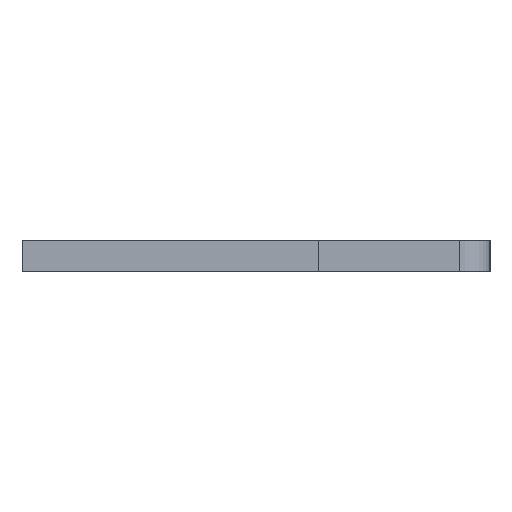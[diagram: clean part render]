
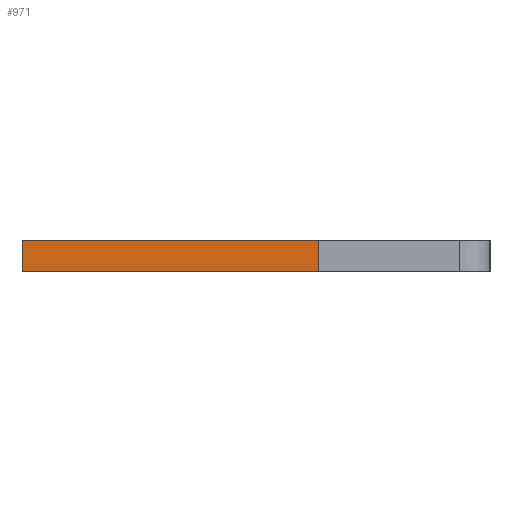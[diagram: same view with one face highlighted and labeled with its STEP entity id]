
A CAD part, left-side view. The second image highlights one B-rep face of the part: STEP entity #971.
In plain terms, the highlighted face is planar.
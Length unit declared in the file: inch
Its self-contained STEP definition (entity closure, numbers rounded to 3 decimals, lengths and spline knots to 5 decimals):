
#16 = LINE ( 'NONE', #1397, #754 ) ;
#61 = ORIENTED_EDGE ( 'NONE', *, *, #1215, .F. ) ;
#216 = ORIENTED_EDGE ( 'NONE', *, *, #1568, .F. ) ;
#306 = CARTESIAN_POINT ( 'NONE',  ( 0.01, 0.15, -0.04 ) ) ;
#328 = CARTESIAN_POINT ( 'NONE',  ( 0.01, 0.15, -0.04 ) ) ;
#353 = VECTOR ( 'NONE', #358, 39.37008 ) ;
#358 = DIRECTION ( 'NONE',  ( -1., 0., 0. ) ) ;
#361 = VERTEX_POINT ( 'NONE', #328 ) ;
#392 = EDGE_CURVE ( 'NONE', #886, #819, #728, .T. ) ;
#464 = CARTESIAN_POINT ( 'NONE',  ( -0.01, 0.15, -0.04 ) ) ;
#503 = VECTOR ( 'NONE', #732, 39.37008 ) ;
#514 = DIRECTION ( 'NONE',  ( 0., 1., 0. ) ) ;
#708 = CARTESIAN_POINT ( 'NONE',  ( 0.01, -0.04, -0.04 ) ) ;
#728 = LINE ( 'NONE', #708, #353 ) ;
#730 = VERTEX_POINT ( 'NONE', #464 ) ;
#732 = DIRECTION ( 'NONE',  ( 0., 1., 0. ) ) ;
#754 = VECTOR ( 'NONE', #514, 39.37008 ) ;
#761 = CARTESIAN_POINT ( 'NONE',  ( -0.01, -0.04, -0.04 ) ) ;
#819 = VERTEX_POINT ( 'NONE', #761 ) ;
#829 = ORIENTED_EDGE ( 'NONE', *, *, #392, .T. ) ;
#834 = DIRECTION ( 'NONE',  ( 0., 0., 1. ) ) ;
#886 = VERTEX_POINT ( 'NONE', #1116 ) ;
#896 = LINE ( 'NONE', #1169, #503 ) ;
#965 = AXIS2_PLACEMENT_3D ( 'NONE', #1416, #834, #1821 ) ;
#971 = ADVANCED_FACE ( 'NONE', ( #1305 ), #1686, .F. ) ;
#1116 = CARTESIAN_POINT ( 'NONE',  ( 0.01, -0.04, -0.04 ) ) ;
#1169 = CARTESIAN_POINT ( 'NONE',  ( -0.01, 0.15, -0.04 ) ) ;
#1215 = EDGE_CURVE ( 'NONE', #886, #361, #16, .T. ) ;
#1305 = FACE_OUTER_BOUND ( 'NONE', #1342, .T. ) ;
#1342 = EDGE_LOOP ( 'NONE', ( #1622, #216, #61, #829 ) ) ;
#1397 = CARTESIAN_POINT ( 'NONE',  ( 0.01, 0.15, -0.04 ) ) ;
#1407 = EDGE_CURVE ( 'NONE', #819, #730, #896, .T. ) ;
#1416 = CARTESIAN_POINT ( 'NONE',  ( 0.01, 0.15, -0.04 ) ) ;
#1513 = LINE ( 'NONE', #306, #1532 ) ;
#1532 = VECTOR ( 'NONE', #1611, 39.37008 ) ;
#1568 = EDGE_CURVE ( 'NONE', #361, #730, #1513, .T. ) ;
#1611 = DIRECTION ( 'NONE',  ( -1., 0., 0. ) ) ;
#1622 = ORIENTED_EDGE ( 'NONE', *, *, #1407, .T. ) ;
#1686 = PLANE ( 'NONE',  #965 ) ;
#1821 = DIRECTION ( 'NONE',  ( 1., 0., 0. ) ) ;
